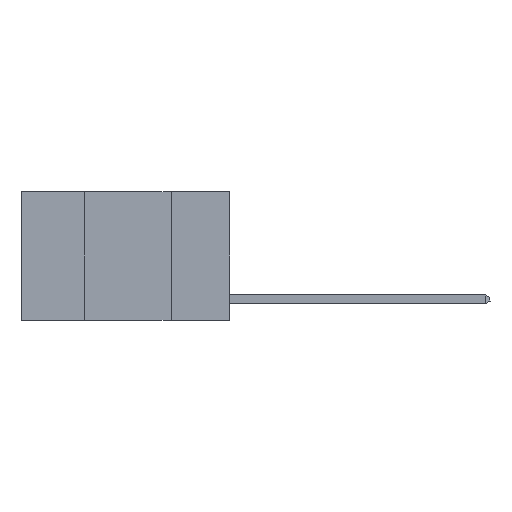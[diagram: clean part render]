
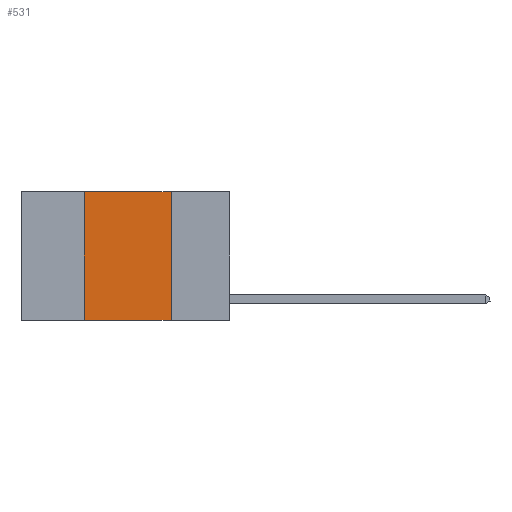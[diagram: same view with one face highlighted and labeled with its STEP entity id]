
A CAD part, left-side view. The second image highlights one B-rep face of the part: STEP entity #531.
In plain terms, the highlighted planar face has unit normal (-1, 0, 0).
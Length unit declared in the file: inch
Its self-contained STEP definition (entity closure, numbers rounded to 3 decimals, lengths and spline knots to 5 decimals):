
#181 = VECTOR ( 'NONE', #7461, 39.37008 ) ;
#190 = EDGE_CURVE ( 'NONE', #7081, #16448, #3942, .T. ) ;
#531 = ADVANCED_FACE ( 'NONE', ( #1460 ), #8822, .F. ) ;
#1066 = CARTESIAN_POINT ( 'NONE',  ( 0., 0.6, 0. ) ) ;
#1458 = DIRECTION ( 'NONE',  ( 0., 0., 1. ) ) ;
#1460 = FACE_OUTER_BOUND ( 'NONE', #9716, .T. ) ;
#1944 = CARTESIAN_POINT ( 'NONE',  ( 0., 0.42, 0. ) ) ;
#2080 = DIRECTION ( 'NONE',  ( 0., 0., -1. ) ) ;
#2537 = ORIENTED_EDGE ( 'NONE', *, *, #14551, .F. ) ;
#3088 = LINE ( 'NONE', #9561, #16776 ) ;
#3442 = CARTESIAN_POINT ( 'NONE',  ( 0., 0.6, 0. ) ) ;
#3942 = LINE ( 'NONE', #13080, #6838 ) ;
#4904 = AXIS2_PLACEMENT_3D ( 'NONE', #3442, #9989, #2080 ) ;
#4931 = DIRECTION ( 'NONE',  ( 0., -1., 0. ) ) ;
#5632 = VECTOR ( 'NONE', #4931, 39.37008 ) ;
#6127 = CARTESIAN_POINT ( 'NONE',  ( 0., 0.17, 0. ) ) ;
#6838 = VECTOR ( 'NONE', #1458, 39.37008 ) ;
#7081 = VERTEX_POINT ( 'NONE', #15554 ) ;
#7461 = DIRECTION ( 'NONE',  ( 0., 0., -1. ) ) ;
#7479 = EDGE_CURVE ( 'NONE', #9255, #9895, #7629, .T. ) ;
#7629 = LINE ( 'NONE', #6127, #181 ) ;
#7830 = EDGE_CURVE ( 'NONE', #7081, #9895, #3088, .T. ) ;
#8822 = PLANE ( 'NONE',  #4904 ) ;
#9255 = VERTEX_POINT ( 'NONE', #15613 ) ;
#9281 = CARTESIAN_POINT ( 'NONE',  ( 0., 0.17, -0.37 ) ) ;
#9561 = CARTESIAN_POINT ( 'NONE',  ( 0., 0.6, -0.37 ) ) ;
#9716 = EDGE_LOOP ( 'NONE', ( #11361, #2537, #10225, #17156 ) ) ;
#9895 = VERTEX_POINT ( 'NONE', #9281 ) ;
#9989 = DIRECTION ( 'NONE',  ( 1., 0., 0. ) ) ;
#10225 = ORIENTED_EDGE ( 'NONE', *, *, #190, .F. ) ;
#10948 = DIRECTION ( 'NONE',  ( 0., -1., 0. ) ) ;
#11361 = ORIENTED_EDGE ( 'NONE', *, *, #7479, .F. ) ;
#12677 = LINE ( 'NONE', #1066, #5632 ) ;
#13080 = CARTESIAN_POINT ( 'NONE',  ( 0., 0.42, 0. ) ) ;
#14551 = EDGE_CURVE ( 'NONE', #16448, #9255, #12677, .T. ) ;
#15554 = CARTESIAN_POINT ( 'NONE',  ( 0., 0.42, -0.37 ) ) ;
#15613 = CARTESIAN_POINT ( 'NONE',  ( 0., 0.17, 0. ) ) ;
#16448 = VERTEX_POINT ( 'NONE', #1944 ) ;
#16776 = VECTOR ( 'NONE', #10948, 39.37008 ) ;
#17156 = ORIENTED_EDGE ( 'NONE', *, *, #7830, .T. ) ;
